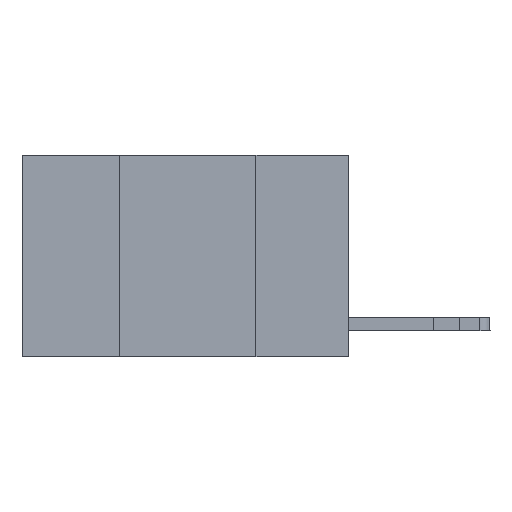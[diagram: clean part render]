
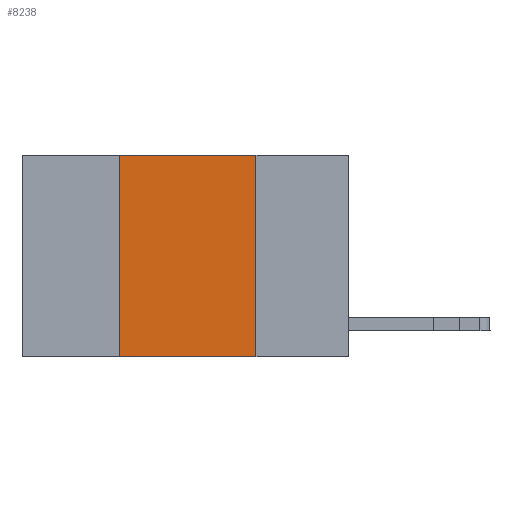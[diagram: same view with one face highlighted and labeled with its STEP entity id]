
A CAD part, left-side view. The second image highlights one B-rep face of the part: STEP entity #8238.
In plain terms, the highlighted planar face has unit normal (-1, 0, 0).
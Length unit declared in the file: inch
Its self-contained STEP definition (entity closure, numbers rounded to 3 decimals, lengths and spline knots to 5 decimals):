
#569 = ORIENTED_EDGE ( 'NONE', *, *, #5112, .F. ) ;
#674 = CARTESIAN_POINT ( 'NONE',  ( 0., 0.17, -0.37 ) ) ;
#836 = ORIENTED_EDGE ( 'NONE', *, *, #7246, .F. ) ;
#875 = DIRECTION ( 'NONE',  ( 0., 0., -1. ) ) ;
#1526 = CARTESIAN_POINT ( 'NONE',  ( 0., 0.42, -0.37 ) ) ;
#1577 = DIRECTION ( 'NONE',  ( 0., -1., 0. ) ) ;
#2193 = DIRECTION ( 'NONE',  ( 0., 0., -1. ) ) ;
#2434 = DIRECTION ( 'NONE',  ( 0., 0., 1. ) ) ;
#2799 = ORIENTED_EDGE ( 'NONE', *, *, #9265, .T. ) ;
#2877 = AXIS2_PLACEMENT_3D ( 'NONE', #6846, #10386, #2193 ) ;
#3359 = CARTESIAN_POINT ( 'NONE',  ( 0., 0.6, -0.37 ) ) ;
#3423 = LINE ( 'NONE', #10885, #4394 ) ;
#3780 = VERTEX_POINT ( 'NONE', #9635 ) ;
#4320 = CARTESIAN_POINT ( 'NONE',  ( 0., 0.42, 0. ) ) ;
#4394 = VECTOR ( 'NONE', #9932, 39.37008 ) ;
#4811 = CARTESIAN_POINT ( 'NONE',  ( 0., 0.17, 0. ) ) ;
#5112 = EDGE_CURVE ( 'NONE', #3780, #8851, #9467, .T. ) ;
#5908 = VERTEX_POINT ( 'NONE', #1526 ) ;
#5996 = VECTOR ( 'NONE', #1577, 39.37008 ) ;
#6846 = CARTESIAN_POINT ( 'NONE',  ( 0., 0.6, 0. ) ) ;
#6991 = LINE ( 'NONE', #3359, #5996 ) ;
#7246 = EDGE_CURVE ( 'NONE', #5908, #9264, #11605, .T. ) ;
#8238 = ADVANCED_FACE ( 'NONE', ( #9689 ), #11298, .F. ) ;
#8851 = VERTEX_POINT ( 'NONE', #674 ) ;
#9212 = ORIENTED_EDGE ( 'NONE', *, *, #11497, .F. ) ;
#9264 = VERTEX_POINT ( 'NONE', #4320 ) ;
#9265 = EDGE_CURVE ( 'NONE', #5908, #8851, #6991, .T. ) ;
#9467 = LINE ( 'NONE', #4811, #11351 ) ;
#9635 = CARTESIAN_POINT ( 'NONE',  ( 0., 0.17, 0. ) ) ;
#9689 = FACE_OUTER_BOUND ( 'NONE', #10419, .T. ) ;
#9932 = DIRECTION ( 'NONE',  ( 0., -1., 0. ) ) ;
#10386 = DIRECTION ( 'NONE',  ( 1., 0., 0. ) ) ;
#10419 = EDGE_LOOP ( 'NONE', ( #569, #9212, #836, #2799 ) ) ;
#10744 = CARTESIAN_POINT ( 'NONE',  ( 0., 0.42, 0. ) ) ;
#10885 = CARTESIAN_POINT ( 'NONE',  ( 0., 0.6, 0. ) ) ;
#11298 = PLANE ( 'NONE',  #2877 ) ;
#11351 = VECTOR ( 'NONE', #875, 39.37008 ) ;
#11497 = EDGE_CURVE ( 'NONE', #9264, #3780, #3423, .T. ) ;
#11605 = LINE ( 'NONE', #10744, #11806 ) ;
#11806 = VECTOR ( 'NONE', #2434, 39.37008 ) ;
